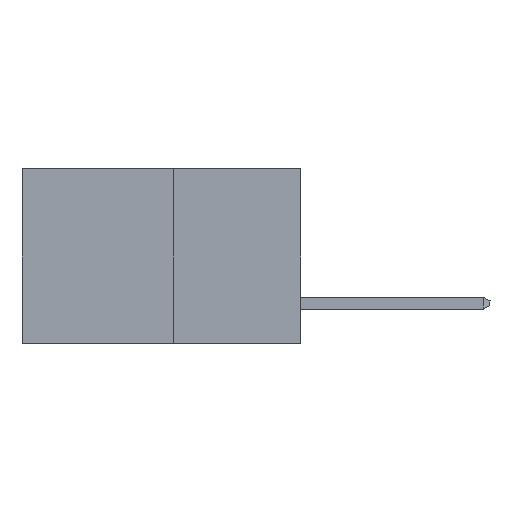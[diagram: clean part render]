
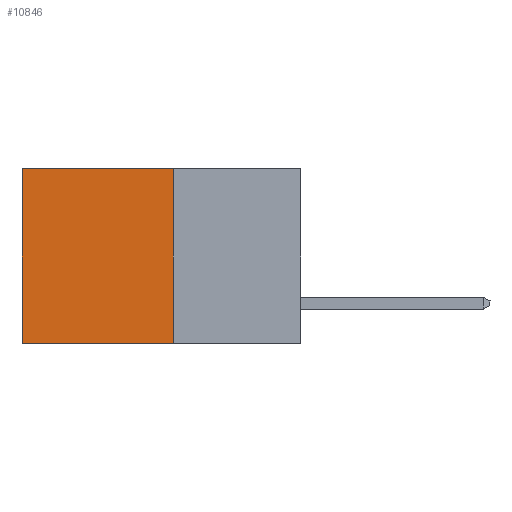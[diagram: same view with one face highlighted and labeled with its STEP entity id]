
A CAD part, left-side view. The second image highlights one B-rep face of the part: STEP entity #10846.
In plain terms, the highlighted planar face has unit normal (-1, 0, 0).
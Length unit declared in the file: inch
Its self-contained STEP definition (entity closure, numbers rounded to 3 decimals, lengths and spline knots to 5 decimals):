
#209 = CARTESIAN_POINT ( 'NONE',  ( 0.277, 0.27, -0.37 ) ) ;
#1557 = CARTESIAN_POINT ( 'NONE',  ( 0.277, 0.27, -0.37 ) ) ;
#2604 = DIRECTION ( 'NONE',  ( 0., 1., 0. ) ) ;
#2747 = DIRECTION ( 'NONE',  ( 0., 0., -1. ) ) ;
#2923 = VECTOR ( 'NONE', #10258, 39.37008 ) ;
#3148 = CARTESIAN_POINT ( 'NONE',  ( 0.277, 0.27, 0. ) ) ;
#3250 = VERTEX_POINT ( 'NONE', #7889 ) ;
#3508 = VECTOR ( 'NONE', #9789, 39.37008 ) ;
#3590 = VERTEX_POINT ( 'NONE', #9876 ) ;
#4006 = VERTEX_POINT ( 'NONE', #10330 ) ;
#4214 = EDGE_CURVE ( 'NONE', #3250, #4006, #8494, .T. ) ;
#5354 = VECTOR ( 'NONE', #2604, 39.37008 ) ;
#5663 = EDGE_LOOP ( 'NONE', ( #7302, #12395, #9820, #7603 ) ) ;
#6009 = EDGE_CURVE ( 'NONE', #3590, #3250, #11552, .T. ) ;
#6105 = PLANE ( 'NONE',  #11605 ) ;
#6461 = EDGE_CURVE ( 'NONE', #3590, #11836, #13672, .T. ) ;
#7302 = ORIENTED_EDGE ( 'NONE', *, *, #8730, .T. ) ;
#7603 = ORIENTED_EDGE ( 'NONE', *, *, #6461, .T. ) ;
#7889 = CARTESIAN_POINT ( 'NONE',  ( 0.277, 0.27, -0.37 ) ) ;
#8494 = LINE ( 'NONE', #11801, #2923 ) ;
#8670 = CARTESIAN_POINT ( 'NONE',  ( 0.277, 0.59, -0.37 ) ) ;
#8730 = EDGE_CURVE ( 'NONE', #11836, #4006, #9423, .T. ) ;
#8825 = CARTESIAN_POINT ( 'NONE',  ( 0.277, 0.59, 0. ) ) ;
#9423 = LINE ( 'NONE', #8670, #3508 ) ;
#9427 = DIRECTION ( 'NONE',  ( 1., 0., 0. ) ) ;
#9789 = DIRECTION ( 'NONE',  ( 0., 0., -1. ) ) ;
#9820 = ORIENTED_EDGE ( 'NONE', *, *, #6009, .F. ) ;
#9876 = CARTESIAN_POINT ( 'NONE',  ( 0.277, 0.27, 0. ) ) ;
#10052 = DIRECTION ( 'NONE',  ( 0., 0., -1. ) ) ;
#10258 = DIRECTION ( 'NONE',  ( 0., 1., 0. ) ) ;
#10330 = CARTESIAN_POINT ( 'NONE',  ( 0.277, 0.59, -0.37 ) ) ;
#10846 = ADVANCED_FACE ( 'NONE', ( #13513 ), #6105, .F. ) ;
#11217 = VECTOR ( 'NONE', #10052, 39.37008 ) ;
#11552 = LINE ( 'NONE', #209, #11217 ) ;
#11605 = AXIS2_PLACEMENT_3D ( 'NONE', #1557, #9427, #2747 ) ;
#11801 = CARTESIAN_POINT ( 'NONE',  ( 0.277, 0.27, -0.37 ) ) ;
#11836 = VERTEX_POINT ( 'NONE', #8825 ) ;
#12395 = ORIENTED_EDGE ( 'NONE', *, *, #4214, .F. ) ;
#13513 = FACE_OUTER_BOUND ( 'NONE', #5663, .T. ) ;
#13672 = LINE ( 'NONE', #3148, #5354 ) ;
